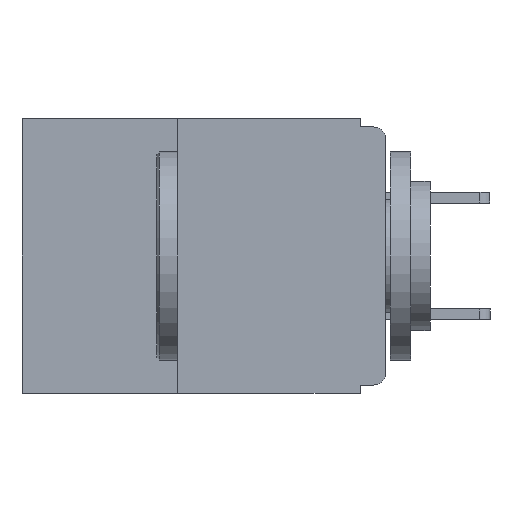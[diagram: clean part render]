
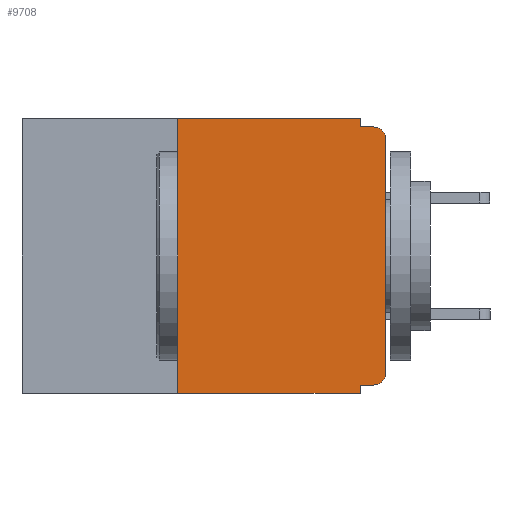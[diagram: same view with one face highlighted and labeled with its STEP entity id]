
A CAD part, left-side view. The second image highlights one B-rep face of the part: STEP entity #9708.
In plain terms, the highlighted planar face has unit normal (-1, 0, 0).
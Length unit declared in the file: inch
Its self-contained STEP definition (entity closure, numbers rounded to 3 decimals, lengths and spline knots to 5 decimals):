
#12 = EDGE_CURVE ( 'NONE', #6049, #5904, #9147, .T. ) ;
#21 = DIRECTION ( 'NONE',  ( 0., -1., 0. ) ) ;
#105 = CARTESIAN_POINT ( 'NONE',  ( 0., 0.25, 0. ) ) ;
#345 = DIRECTION ( 'NONE',  ( -1., 0., 0. ) ) ;
#409 = VERTEX_POINT ( 'NONE', #105 ) ;
#411 = EDGE_CURVE ( 'NONE', #16557, #409, #5709, .T. ) ;
#626 = EDGE_CURVE ( 'NONE', #409, #7797, #3456, .T. ) ;
#1091 = VECTOR ( 'NONE', #12468, 39.37008 ) ;
#1556 = LINE ( 'NONE', #12857, #1091 ) ;
#1767 = VECTOR ( 'NONE', #5940, 39.37008 ) ;
#1834 = VECTOR ( 'NONE', #15295, 39.37008 ) ;
#2135 = VECTOR ( 'NONE', #6446, 39.37008 ) ;
#2187 = AXIS2_PLACEMENT_3D ( 'NONE', #17998, #17994, #17974 ) ;
#2225 = VERTEX_POINT ( 'NONE', #6599 ) ;
#2713 = DIRECTION ( 'NONE',  ( 0., -1., 0. ) ) ;
#2716 = CARTESIAN_POINT ( 'NONE',  ( 0., 0.437, 0. ) ) ;
#2795 = DIRECTION ( 'NONE',  ( 0., -1., 0. ) ) ;
#3013 = VECTOR ( 'NONE', #2713, 39.37008 ) ;
#3226 = CARTESIAN_POINT ( 'NONE',  ( 0., 0.015, -0.025 ) ) ;
#3456 = LINE ( 'NONE', #2716, #3013 ) ;
#3744 = EDGE_CURVE ( 'NONE', #5904, #2225, #5990, .T. ) ;
#4375 = EDGE_CURVE ( 'NONE', #16557, #6940, #14947, .T. ) ;
#4651 = DIRECTION ( 'NONE',  ( 0., 0., -1. ) ) ;
#4906 = VECTOR ( 'NONE', #6223, 39.37008 ) ;
#4915 = ORIENTED_EDGE ( 'NONE', *, *, #3744, .T. ) ;
#5059 = CARTESIAN_POINT ( 'NONE',  ( 0., 0.437, -0.33 ) ) ;
#5180 = CARTESIAN_POINT ( 'NONE',  ( 0., 0., 0. ) ) ;
#5639 = LINE ( 'NONE', #8789, #1767 ) ;
#5709 = LINE ( 'NONE', #12491, #1834 ) ;
#5904 = VERTEX_POINT ( 'NONE', #8215 ) ;
#5940 = DIRECTION ( 'NONE',  ( 0., 0., -1. ) ) ;
#5964 = FACE_OUTER_BOUND ( 'NONE', #15722, .T. ) ;
#5990 = LINE ( 'NONE', #5180, #2135 ) ;
#6049 = VERTEX_POINT ( 'NONE', #17800 ) ;
#6181 = VERTEX_POINT ( 'NONE', #15377 ) ;
#6223 = DIRECTION ( 'NONE',  ( 0., 1., 0. ) ) ;
#6266 = CARTESIAN_POINT ( 'NONE',  ( 0., 0., -0.32 ) ) ;
#6282 = DIRECTION ( 'NONE',  ( 0., 0., -1. ) ) ;
#6325 = EDGE_CURVE ( 'NONE', #13733, #6940, #1556, .T. ) ;
#6446 = DIRECTION ( 'NONE',  ( 0., 0., 1. ) ) ;
#6599 = CARTESIAN_POINT ( 'NONE',  ( 0., 0., -0.025 ) ) ;
#6940 = VERTEX_POINT ( 'NONE', #17562 ) ;
#7387 = VERTEX_POINT ( 'NONE', #13710 ) ;
#7797 = VERTEX_POINT ( 'NONE', #10145 ) ;
#8215 = CARTESIAN_POINT ( 'NONE',  ( 0., 0., -0.305 ) ) ;
#8250 = EDGE_CURVE ( 'NONE', #6049, #13733, #9226, .T. ) ;
#8789 = CARTESIAN_POINT ( 'NONE',  ( 0., 0.031, 0. ) ) ;
#9010 = ORIENTED_EDGE ( 'NONE', *, *, #8250, .F. ) ;
#9147 = CIRCLE ( 'NONE', #15894, 0.015 ) ;
#9226 = LINE ( 'NONE', #6266, #4906 ) ;
#9440 = ORIENTED_EDGE ( 'NONE', *, *, #6325, .F. ) ;
#9708 = ADVANCED_FACE ( 'NONE', ( #5964 ), #18158, .F. ) ;
#9951 = VECTOR ( 'NONE', #21, 39.37008 ) ;
#10145 = CARTESIAN_POINT ( 'NONE',  ( 0., 0.031, 0. ) ) ;
#10463 = CARTESIAN_POINT ( 'NONE',  ( 0., 0.031, -0.32 ) ) ;
#11179 = VECTOR ( 'NONE', #2795, 39.37008 ) ;
#12370 = ORIENTED_EDGE ( 'NONE', *, *, #4375, .T. ) ;
#12468 = DIRECTION ( 'NONE',  ( 0., 0., -1. ) ) ;
#12491 = CARTESIAN_POINT ( 'NONE',  ( 0., 0.25, -0.33 ) ) ;
#12857 = CARTESIAN_POINT ( 'NONE',  ( 0., 0.031, -0.33 ) ) ;
#13049 = EDGE_CURVE ( 'NONE', #2225, #6181, #17185, .T. ) ;
#13054 = CARTESIAN_POINT ( 'NONE',  ( 0., 0., -0.01 ) ) ;
#13273 = CARTESIAN_POINT ( 'NONE',  ( 0., 0.25, -0.33 ) ) ;
#13299 = DIRECTION ( 'NONE',  ( -1., 0., 0. ) ) ;
#13710 = CARTESIAN_POINT ( 'NONE',  ( 0., 0.031, -0.01 ) ) ;
#13733 = VERTEX_POINT ( 'NONE', #10463 ) ;
#13764 = LINE ( 'NONE', #13054, #9951 ) ;
#14901 = AXIS2_PLACEMENT_3D ( 'NONE', #3226, #13299, #4651 ) ;
#14927 = ORIENTED_EDGE ( 'NONE', *, *, #411, .F. ) ;
#14947 = LINE ( 'NONE', #5059, #11179 ) ;
#15287 = ORIENTED_EDGE ( 'NONE', *, *, #626, .F. ) ;
#15295 = DIRECTION ( 'NONE',  ( 0., 0., 1. ) ) ;
#15377 = CARTESIAN_POINT ( 'NONE',  ( 0., 0.015, -0.01 ) ) ;
#15722 = EDGE_LOOP ( 'NONE', ( #4915, #16289, #16673, #16929, #15287, #14927, #12370, #9440, #9010, #16323 ) ) ;
#15894 = AXIS2_PLACEMENT_3D ( 'NONE', #16009, #345, #6282 ) ;
#16009 = CARTESIAN_POINT ( 'NONE',  ( 0., 0.015, -0.305 ) ) ;
#16289 = ORIENTED_EDGE ( 'NONE', *, *, #13049, .T. ) ;
#16323 = ORIENTED_EDGE ( 'NONE', *, *, #12, .T. ) ;
#16557 = VERTEX_POINT ( 'NONE', #13273 ) ;
#16673 = ORIENTED_EDGE ( 'NONE', *, *, #17104, .F. ) ;
#16929 = ORIENTED_EDGE ( 'NONE', *, *, #17130, .F. ) ;
#17104 = EDGE_CURVE ( 'NONE', #7387, #6181, #13764, .T. ) ;
#17130 = EDGE_CURVE ( 'NONE', #7797, #7387, #5639, .T. ) ;
#17185 = CIRCLE ( 'NONE', #14901, 0.015 ) ;
#17562 = CARTESIAN_POINT ( 'NONE',  ( 0., 0.031, -0.33 ) ) ;
#17800 = CARTESIAN_POINT ( 'NONE',  ( 0., 0.015, -0.32 ) ) ;
#17974 = DIRECTION ( 'NONE',  ( 0., 0., -1. ) ) ;
#17994 = DIRECTION ( 'NONE',  ( 1., 0., 0. ) ) ;
#17998 = CARTESIAN_POINT ( 'NONE',  ( 0., 0.437, 0. ) ) ;
#18158 = PLANE ( 'NONE',  #2187 ) ;
